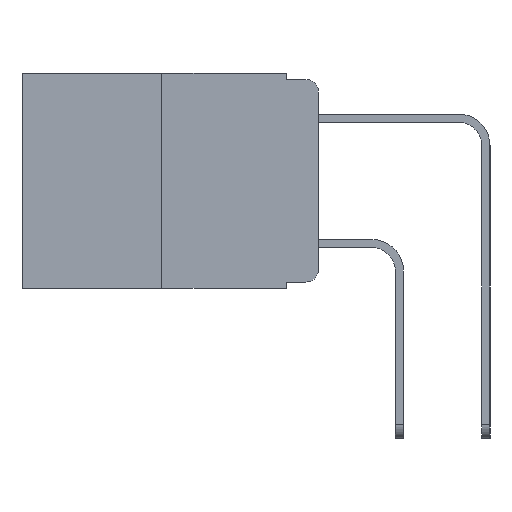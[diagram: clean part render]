
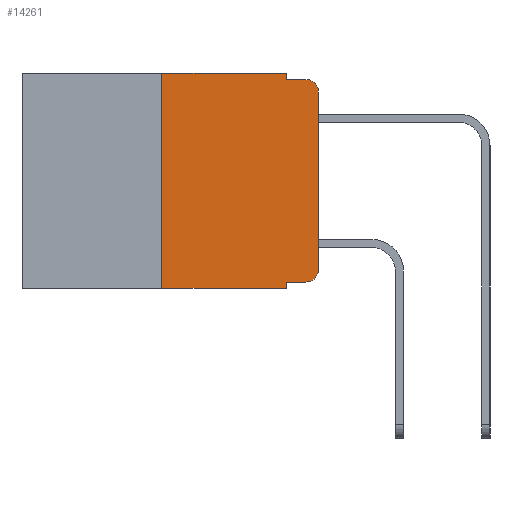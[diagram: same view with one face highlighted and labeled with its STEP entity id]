
A CAD part, left-side view. The second image highlights one B-rep face of the part: STEP entity #14261.
In plain terms, the highlighted planar face has unit normal (-1, 0, 0).
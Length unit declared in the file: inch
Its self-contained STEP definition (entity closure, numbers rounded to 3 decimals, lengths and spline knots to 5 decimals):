
#17 = LINE ( 'NONE', #11577, #15387 ) ;
#29 = EDGE_CURVE ( 'NONE', #8896, #15882, #7953, .T. ) ;
#96 = LINE ( 'NONE', #3726, #7957 ) ;
#311 = CARTESIAN_POINT ( 'NONE',  ( 0., 0., 0. ) ) ;
#357 = CARTESIAN_POINT ( 'NONE',  ( 0., 0.473, 0. ) ) ;
#1143 = AXIS2_PLACEMENT_3D ( 'NONE', #1489, #2148, #2117 ) ;
#1311 = VERTEX_POINT ( 'NONE', #19505 ) ;
#1395 = CARTESIAN_POINT ( 'NONE',  ( 0., 0.473, -0.343 ) ) ;
#1489 = CARTESIAN_POINT ( 'NONE',  ( 0., 0.02, -0.03 ) ) ;
#1697 = DIRECTION ( 'NONE',  ( 0., -1., 0. ) ) ;
#1890 = DIRECTION ( 'NONE',  ( 0., 0., 1. ) ) ;
#1892 = EDGE_CURVE ( 'NONE', #1311, #4437, #8216, .T. ) ;
#1928 = DIRECTION ( 'NONE',  ( 1., 0., 0. ) ) ;
#2117 = DIRECTION ( 'NONE',  ( 0., 0., -1. ) ) ;
#2143 = VECTOR ( 'NONE', #17908, 39.37008 ) ;
#2148 = DIRECTION ( 'NONE',  ( -1., 0., 0. ) ) ;
#2975 = EDGE_CURVE ( 'NONE', #10008, #3719, #17250, .T. ) ;
#3290 = DIRECTION ( 'NONE',  ( 0., -1., 0. ) ) ;
#3520 = ORIENTED_EDGE ( 'NONE', *, *, #13634, .T. ) ;
#3719 = VERTEX_POINT ( 'NONE', #17015 ) ;
#3726 = CARTESIAN_POINT ( 'NONE',  ( 0., 0.051, 0. ) ) ;
#3845 = ORIENTED_EDGE ( 'NONE', *, *, #6539, .F. ) ;
#4117 = ORIENTED_EDGE ( 'NONE', *, *, #29, .F. ) ;
#4326 = CARTESIAN_POINT ( 'NONE',  ( 0., 0.473, 0. ) ) ;
#4436 = CARTESIAN_POINT ( 'NONE',  ( 0., 0.051, -0.333 ) ) ;
#4437 = VERTEX_POINT ( 'NONE', #5291 ) ;
#4741 = CARTESIAN_POINT ( 'NONE',  ( 0., 0.051, -0.333 ) ) ;
#4761 = EDGE_CURVE ( 'NONE', #3719, #6631, #18347, .T. ) ;
#4791 = ORIENTED_EDGE ( 'NONE', *, *, #13275, .F. ) ;
#4854 = ORIENTED_EDGE ( 'NONE', *, *, #2975, .T. ) ;
#5003 = VERTEX_POINT ( 'NONE', #9651 ) ;
#5291 = CARTESIAN_POINT ( 'NONE',  ( 0., 0.02, -0.01 ) ) ;
#5326 = VECTOR ( 'NONE', #1697, 39.37008 ) ;
#6122 = EDGE_LOOP ( 'NONE', ( #3520, #10343, #7685, #6320, #4117, #3845, #6704, #4791, #4854, #11383 ) ) ;
#6320 = ORIENTED_EDGE ( 'NONE', *, *, #17546, .F. ) ;
#6539 = EDGE_CURVE ( 'NONE', #8704, #8896, #14557, .T. ) ;
#6631 = VERTEX_POINT ( 'NONE', #16044 ) ;
#6704 = ORIENTED_EDGE ( 'NONE', *, *, #18495, .T. ) ;
#7144 = LINE ( 'NONE', #311, #17162 ) ;
#7370 = VECTOR ( 'NONE', #3290, 39.37008 ) ;
#7685 = ORIENTED_EDGE ( 'NONE', *, *, #19247, .F. ) ;
#7953 = LINE ( 'NONE', #4326, #7370 ) ;
#7957 = VECTOR ( 'NONE', #8408, 39.37008 ) ;
#8081 = CARTESIAN_POINT ( 'NONE',  ( 0., 0.051, -0.343 ) ) ;
#8216 = CIRCLE ( 'NONE', #1143, 0.02 ) ;
#8408 = DIRECTION ( 'NONE',  ( 0., 0., -1. ) ) ;
#8518 = AXIS2_PLACEMENT_3D ( 'NONE', #12916, #12846, #12364 ) ;
#8704 = VERTEX_POINT ( 'NONE', #9135 ) ;
#8896 = VERTEX_POINT ( 'NONE', #15593 ) ;
#9135 = CARTESIAN_POINT ( 'NONE',  ( 0., 0.25, -0.343 ) ) ;
#9651 = CARTESIAN_POINT ( 'NONE',  ( 0., 0.051, -0.01 ) ) ;
#10008 = VERTEX_POINT ( 'NONE', #4741 ) ;
#10141 = DIRECTION ( 'NONE',  ( 0., 0., -1. ) ) ;
#10343 = ORIENTED_EDGE ( 'NONE', *, *, #1892, .T. ) ;
#10525 = VECTOR ( 'NONE', #10704, 39.37008 ) ;
#10704 = DIRECTION ( 'NONE',  ( 0., -1., 0. ) ) ;
#10839 = VERTEX_POINT ( 'NONE', #8081 ) ;
#10913 = AXIS2_PLACEMENT_3D ( 'NONE', #357, #1928, #12725 ) ;
#11383 = ORIENTED_EDGE ( 'NONE', *, *, #4761, .T. ) ;
#11577 = CARTESIAN_POINT ( 'NONE',  ( 0., 0.051, 0. ) ) ;
#12364 = DIRECTION ( 'NONE',  ( 0., 0., -1. ) ) ;
#12725 = DIRECTION ( 'NONE',  ( 0., 0., -1. ) ) ;
#12846 = DIRECTION ( 'NONE',  ( -1., 0., 0. ) ) ;
#12916 = CARTESIAN_POINT ( 'NONE',  ( 0., 0.02, -0.313 ) ) ;
#13275 = EDGE_CURVE ( 'NONE', #10008, #10839, #17, .T. ) ;
#13634 = EDGE_CURVE ( 'NONE', #6631, #1311, #7144, .T. ) ;
#13913 = DIRECTION ( 'NONE',  ( 0., 0., 1. ) ) ;
#14090 = VECTOR ( 'NONE', #13913, 39.37008 ) ;
#14204 = CARTESIAN_POINT ( 'NONE',  ( 0., 0.25, 0. ) ) ;
#14261 = ADVANCED_FACE ( 'NONE', ( #14432 ), #18547, .F. ) ;
#14399 = LINE ( 'NONE', #16448, #2143 ) ;
#14432 = FACE_OUTER_BOUND ( 'NONE', #6122, .T. ) ;
#14514 = LINE ( 'NONE', #1395, #10525 ) ;
#14557 = LINE ( 'NONE', #14204, #14090 ) ;
#15387 = VECTOR ( 'NONE', #10141, 39.37008 ) ;
#15593 = CARTESIAN_POINT ( 'NONE',  ( 0., 0.25, 0. ) ) ;
#15882 = VERTEX_POINT ( 'NONE', #18046 ) ;
#16044 = CARTESIAN_POINT ( 'NONE',  ( 0., 0., -0.313 ) ) ;
#16448 = CARTESIAN_POINT ( 'NONE',  ( 0., 0.051, -0.01 ) ) ;
#17015 = CARTESIAN_POINT ( 'NONE',  ( 0., 0.02, -0.333 ) ) ;
#17162 = VECTOR ( 'NONE', #1890, 39.37008 ) ;
#17250 = LINE ( 'NONE', #4436, #5326 ) ;
#17546 = EDGE_CURVE ( 'NONE', #15882, #5003, #96, .T. ) ;
#17908 = DIRECTION ( 'NONE',  ( 0., -1., 0. ) ) ;
#18046 = CARTESIAN_POINT ( 'NONE',  ( 0., 0.051, 0. ) ) ;
#18347 = CIRCLE ( 'NONE', #8518, 0.02 ) ;
#18495 = EDGE_CURVE ( 'NONE', #8704, #10839, #14514, .T. ) ;
#18547 = PLANE ( 'NONE',  #10913 ) ;
#19247 = EDGE_CURVE ( 'NONE', #5003, #4437, #14399, .T. ) ;
#19505 = CARTESIAN_POINT ( 'NONE',  ( 0., 0., -0.03 ) ) ;
